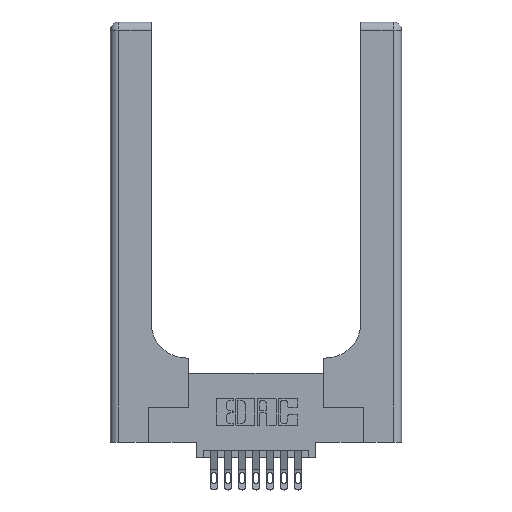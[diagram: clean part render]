
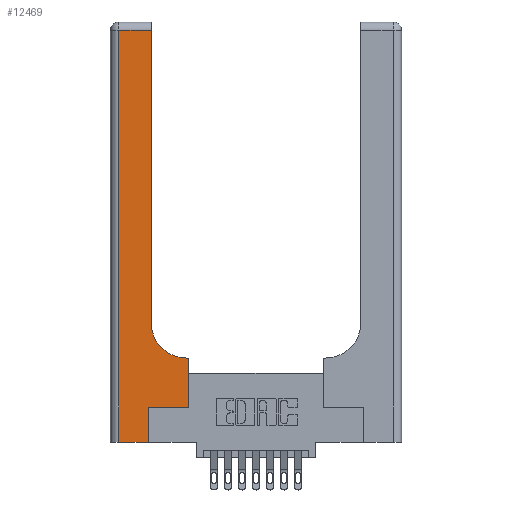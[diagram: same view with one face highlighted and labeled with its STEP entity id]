
A CAD part, top view. The second image highlights one B-rep face of the part: STEP entity #12469.
In plain terms, the highlighted planar face has unit normal (0, 0, 1).
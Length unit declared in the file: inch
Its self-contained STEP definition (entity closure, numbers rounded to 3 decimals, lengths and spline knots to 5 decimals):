
#15 = CARTESIAN_POINT ( 'NONE',  ( 0.06, 3., 0.37 ) ) ;
#112 = PLANE ( 'NONE',  #3597 ) ;
#343 = CARTESIAN_POINT ( 'NONE',  ( 0.2915, 0.6, 0.37 ) ) ;
#478 = DIRECTION ( 'NONE',  ( -1., 0., 0. ) ) ;
#588 = ORIENTED_EDGE ( 'NONE', *, *, #6551, .T. ) ;
#818 = CIRCLE ( 'NONE', #4827, 0.25 ) ;
#997 = DIRECTION ( 'NONE',  ( 1., 0., 0. ) ) ;
#1244 = DIRECTION ( 'NONE',  ( 0., -1., 0. ) ) ;
#1292 = CARTESIAN_POINT ( 'NONE',  ( 0., 3., 0.37 ) ) ;
#1295 = VERTEX_POINT ( 'NONE', #2255 ) ;
#1583 = EDGE_CURVE ( 'NONE', #15078, #4415, #9440, .T. ) ;
#2213 = VECTOR ( 'NONE', #2309, 39.37008 ) ;
#2255 = CARTESIAN_POINT ( 'NONE',  ( 0.06, 0., 0.37 ) ) ;
#2309 = DIRECTION ( 'NONE',  ( 0., 1., 0. ) ) ;
#2604 = VECTOR ( 'NONE', #3937, 39.37008 ) ;
#2622 = ORIENTED_EDGE ( 'NONE', *, *, #9839, .T. ) ;
#3162 = CARTESIAN_POINT ( 'NONE',  ( 0.5415, 0.6, 0.37 ) ) ;
#3458 = DIRECTION ( 'NONE',  ( 1., 0., 0. ) ) ;
#3597 = AXIS2_PLACEMENT_3D ( 'NONE', #1292, #7443, #9708 ) ;
#3937 = DIRECTION ( 'NONE',  ( 1., 0., 0. ) ) ;
#4150 = EDGE_CURVE ( 'NONE', #8538, #1295, #14377, .T. ) ;
#4415 = VERTEX_POINT ( 'NONE', #14937 ) ;
#4827 = AXIS2_PLACEMENT_3D ( 'NONE', #5822, #8303, #3458 ) ;
#4905 = VECTOR ( 'NONE', #8999, 39.37008 ) ;
#4982 = VECTOR ( 'NONE', #14695, 39.37008 ) ;
#5285 = LINE ( 'NONE', #13738, #4905 ) ;
#5471 = LINE ( 'NONE', #14673, #2213 ) ;
#5536 = EDGE_CURVE ( 'NONE', #6546, #15078, #11432, .T. ) ;
#5821 = EDGE_CURVE ( 'NONE', #6213, #8538, #9135, .T. ) ;
#5822 = CARTESIAN_POINT ( 'NONE',  ( 0.5415, 0.85, 0.37 ) ) ;
#5931 = CARTESIAN_POINT ( 'NONE',  ( 0.269, 0.25, 0.37 ) ) ;
#5955 = VERTEX_POINT ( 'NONE', #15096 ) ;
#6213 = VERTEX_POINT ( 'NONE', #14295 ) ;
#6546 = VERTEX_POINT ( 'NONE', #7675 ) ;
#6551 = EDGE_CURVE ( 'NONE', #5955, #12864, #14506, .T. ) ;
#6637 = CARTESIAN_POINT ( 'NONE',  ( 0.06, 2.94, 0.37 ) ) ;
#7321 = EDGE_CURVE ( 'NONE', #4415, #5955, #5285, .T. ) ;
#7368 = ORIENTED_EDGE ( 'NONE', *, *, #11232, .T. ) ;
#7412 = CARTESIAN_POINT ( 'NONE',  ( 0.269, 0., 0.37 ) ) ;
#7443 = DIRECTION ( 'NONE',  ( 0., 0., -1. ) ) ;
#7675 = CARTESIAN_POINT ( 'NONE',  ( 0.269, 0., 0.37 ) ) ;
#7746 = VERTEX_POINT ( 'NONE', #10810 ) ;
#8303 = DIRECTION ( 'NONE',  ( 0., 0., -1. ) ) ;
#8538 = VERTEX_POINT ( 'NONE', #6637 ) ;
#8872 = LINE ( 'NONE', #15097, #2604 ) ;
#8880 = DIRECTION ( 'NONE',  ( -1., 0., 0. ) ) ;
#8999 = DIRECTION ( 'NONE',  ( 0., 1., 0. ) ) ;
#9135 = LINE ( 'NONE', #11219, #14909 ) ;
#9419 = ORIENTED_EDGE ( 'NONE', *, *, #7321, .T. ) ;
#9440 = LINE ( 'NONE', #5931, #14251 ) ;
#9708 = DIRECTION ( 'NONE',  ( -1., 0., 0. ) ) ;
#9817 = ORIENTED_EDGE ( 'NONE', *, *, #4150, .T. ) ;
#9839 = EDGE_CURVE ( 'NONE', #1295, #6546, #8872, .T. ) ;
#10088 = ORIENTED_EDGE ( 'NONE', *, *, #15344, .T. ) ;
#10274 = CARTESIAN_POINT ( 'NONE',  ( 0.269, 0.25, 0.37 ) ) ;
#10524 = FACE_OUTER_BOUND ( 'NONE', #12006, .T. ) ;
#10810 = CARTESIAN_POINT ( 'NONE',  ( 0.2915, 0.85, 0.37 ) ) ;
#11083 = VECTOR ( 'NONE', #1244, 39.37008 ) ;
#11219 = CARTESIAN_POINT ( 'NONE',  ( 0., 2.94, 0.37 ) ) ;
#11232 = EDGE_CURVE ( 'NONE', #12864, #7746, #818, .T. ) ;
#11432 = LINE ( 'NONE', #7412, #4982 ) ;
#11592 = VECTOR ( 'NONE', #8880, 39.37008 ) ;
#12006 = EDGE_LOOP ( 'NONE', ( #10088, #15720, #9817, #2622, #12549, #13461, #9419, #588, #7368 ) ) ;
#12469 = ADVANCED_FACE ( 'NONE', ( #10524 ), #112, .F. ) ;
#12549 = ORIENTED_EDGE ( 'NONE', *, *, #5536, .T. ) ;
#12864 = VERTEX_POINT ( 'NONE', #3162 ) ;
#13461 = ORIENTED_EDGE ( 'NONE', *, *, #1583, .T. ) ;
#13738 = CARTESIAN_POINT ( 'NONE',  ( 0.5585, 0.25, 0.37 ) ) ;
#14251 = VECTOR ( 'NONE', #997, 39.37008 ) ;
#14295 = CARTESIAN_POINT ( 'NONE',  ( 0.2915, 2.94, 0.37 ) ) ;
#14377 = LINE ( 'NONE', #15, #11083 ) ;
#14506 = LINE ( 'NONE', #343, #11592 ) ;
#14673 = CARTESIAN_POINT ( 'NONE',  ( 0.2915, 3., 0.37 ) ) ;
#14695 = DIRECTION ( 'NONE',  ( 0., 1., 0. ) ) ;
#14909 = VECTOR ( 'NONE', #478, 39.37008 ) ;
#14937 = CARTESIAN_POINT ( 'NONE',  ( 0.5585, 0.25, 0.37 ) ) ;
#15078 = VERTEX_POINT ( 'NONE', #10274 ) ;
#15096 = CARTESIAN_POINT ( 'NONE',  ( 0.5585, 0.6, 0.37 ) ) ;
#15097 = CARTESIAN_POINT ( 'NONE',  ( 0., 0., 0.37 ) ) ;
#15344 = EDGE_CURVE ( 'NONE', #7746, #6213, #5471, .T. ) ;
#15720 = ORIENTED_EDGE ( 'NONE', *, *, #5821, .T. ) ;
